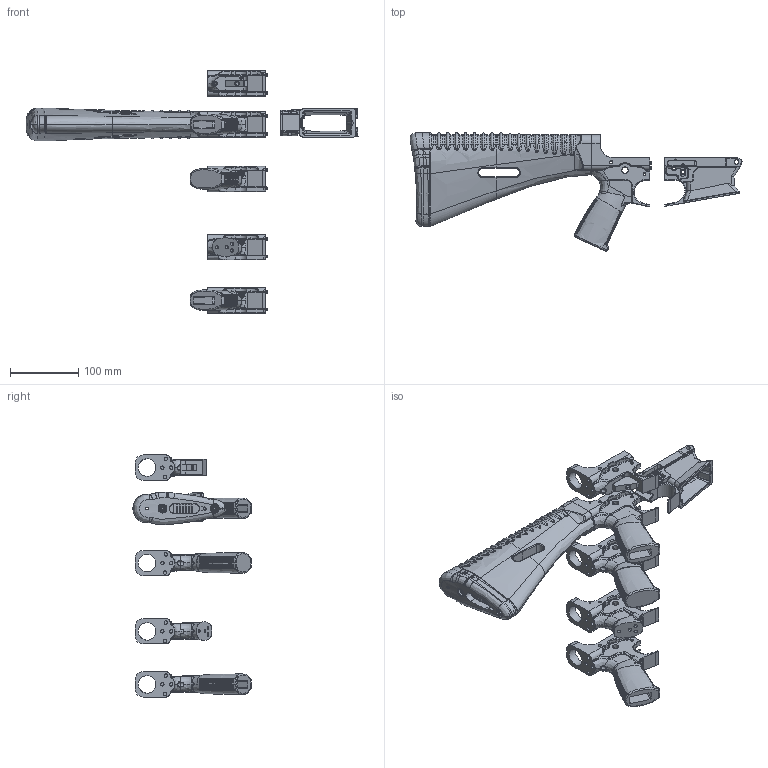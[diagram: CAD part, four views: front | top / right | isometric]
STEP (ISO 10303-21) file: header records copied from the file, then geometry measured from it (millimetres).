
FILE_DESCRIPTION(/* description */ (''),/* implementation_level */ '2;1');
FILE_NAME(/* name */ 'AA1 v12.step',/* time_stamp */ '2020-05-20T22:26:06-05:00',/* author */ (''),/* organization */ (''),/* preprocessor_version */ 'ST-DEVELOPER v18.1',/* originating_system */ 'Autodesk Translation Framework v9.3.0.1241',/* authorisation */ '');
FILE_SCHEMA (('AUTOMOTIVE_DESIGN { 1 0 10303 214 3 1 1 }'));
Products named in the file (1): AA1
Bounding box: 486.69 x 173.26 x 354.93 mm (x, y, z)
Volume: 1421344.7 mm3; surface area: 351381.1 mm2
Topology: 13 solids, 25 shells, 4267 faces, 11964 edges, 7820 vertices
Faces by surface type: plane 1598, bspline 1475, cylinder 836, torus 313, sphere 33, cone 12
Full cylindrical faces by diameter (mm): 2 x2, 2.103 x1, 2.362 x2, 3 x3, 3.175 x13, 3.2 x4, 3.5 x2, 3.945 x3, 3.962 x2, 3.969 x11, 4 x18, 4.238 x6, 4.317 x4, 4.826 x9, 4.9 x1, 5 x36, 5.08 x4, 5.182 x1, 5.389 x1, 5.394 x1, 5.436 x2, 5.596 x2, 5.687 x2, 6.375 x2, 6.477 x5, 6.502 x1, 6.858 x2, 7.036 x3, 7.06 x2, 7.938 x1
Entity records: 289520 total; most frequent: CARTESIAN_POINT 192195, ORIENTED_EDGE 23886, DIRECTION 14896, EDGE_CURVE 11943, VERTEX_POINT 7830, AXIS2_PLACEMENT_3D 5607, B_SPLINE_CURVE_WITH_KNOTS 5420, EDGE_LOOP 4527
